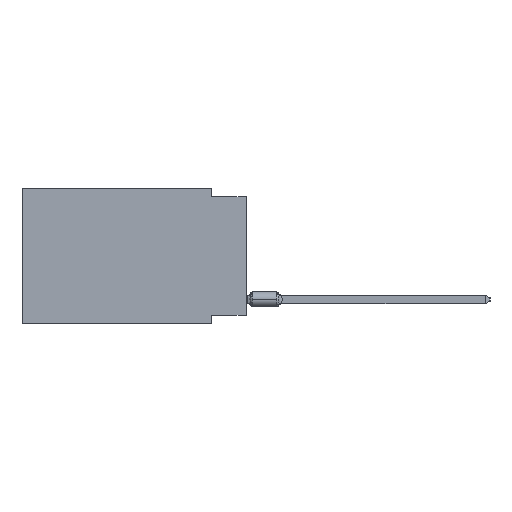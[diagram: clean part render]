
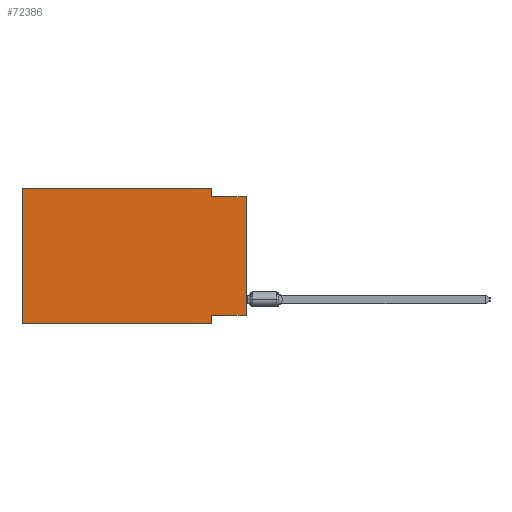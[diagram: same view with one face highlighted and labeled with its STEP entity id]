
A CAD part, left-side view. The second image highlights one B-rep face of the part: STEP entity #72386.
In plain terms, the highlighted planar face has unit normal (-1, 0, 0).
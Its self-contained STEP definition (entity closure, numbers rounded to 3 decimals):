
#480 = EDGE_CURVE ( 'NONE', #50530, #59413, #16337, .T. ) ;
#1245 = VERTEX_POINT ( 'NONE', #71798 ) ;
#3922 = VECTOR ( 'NONE', #43451, 1000. ) ;
#4442 = DIRECTION ( 'NONE',  ( 0., -1., 0. ) ) ;
#7585 = DIRECTION ( 'NONE',  ( 0., 1., 0. ) ) ;
#7791 = VECTOR ( 'NONE', #7585, 1000. ) ;
#11571 = CARTESIAN_POINT ( 'NONE',  ( 0., 16.383, -9.906 ) ) ;
#12327 = PLANE ( 'NONE',  #35123 ) ;
#13555 = CARTESIAN_POINT ( 'NONE',  ( 0., 16.383, -9.906 ) ) ;
#14518 = DIRECTION ( 'NONE',  ( 0., 0., 1. ) ) ;
#15463 = CARTESIAN_POINT ( 'NONE',  ( 0., 16.383, 0. ) ) ;
#16337 = LINE ( 'NONE', #63091, #64548 ) ;
#17380 = CARTESIAN_POINT ( 'NONE',  ( 0., 16.383, 0. ) ) ;
#17696 = EDGE_CURVE ( 'NONE', #68012, #49592, #25215, .T. ) ;
#18709 = CARTESIAN_POINT ( 'NONE',  ( 0., 0., -9.271 ) ) ;
#20062 = CARTESIAN_POINT ( 'NONE',  ( 0., 2.54, -9.906 ) ) ;
#20744 = CARTESIAN_POINT ( 'NONE',  ( 0., 2.54, -9.271 ) ) ;
#21152 = VECTOR ( 'NONE', #14518, 1000. ) ;
#22748 = DIRECTION ( 'NONE',  ( 0., -1., 0. ) ) ;
#22846 = ORIENTED_EDGE ( 'NONE', *, *, #22960, .T. ) ;
#22960 = EDGE_CURVE ( 'NONE', #47992, #1245, #29202, .T. ) ;
#25215 = LINE ( 'NONE', #18709, #7791 ) ;
#25536 = LINE ( 'NONE', #48915, #47731 ) ;
#25605 = LINE ( 'NONE', #72354, #75083 ) ;
#25841 = VERTEX_POINT ( 'NONE', #29473 ) ;
#29111 = EDGE_CURVE ( 'NONE', #39695, #25841, #40395, .T. ) ;
#29202 = LINE ( 'NONE', #11571, #71847 ) ;
#29473 = CARTESIAN_POINT ( 'NONE',  ( 0., 2.54, 0. ) ) ;
#31081 = CARTESIAN_POINT ( 'NONE',  ( 0., 2.54, -0.635 ) ) ;
#31616 = ORIENTED_EDGE ( 'NONE', *, *, #41038, .T. ) ;
#31671 = ORIENTED_EDGE ( 'NONE', *, *, #480, .F. ) ;
#33798 = ORIENTED_EDGE ( 'NONE', *, *, #29111, .F. ) ;
#35123 = AXIS2_PLACEMENT_3D ( 'NONE', #70969, #59468, #35718 ) ;
#35718 = DIRECTION ( 'NONE',  ( 0., 0., -1. ) ) ;
#37394 = VECTOR ( 'NONE', #22748, 1000. ) ;
#39695 = VERTEX_POINT ( 'NONE', #15463 ) ;
#39713 = EDGE_CURVE ( 'NONE', #49592, #1245, #72571, .T. ) ;
#40395 = LINE ( 'NONE', #17380, #37394 ) ;
#40529 = EDGE_CURVE ( 'NONE', #47992, #39695, #61673, .T. ) ;
#41038 = EDGE_CURVE ( 'NONE', #68012, #59413, #25536, .T. ) ;
#43451 = DIRECTION ( 'NONE',  ( 0., 0., -1. ) ) ;
#45725 = DIRECTION ( 'NONE',  ( 0., -1., 0. ) ) ;
#46124 = ORIENTED_EDGE ( 'NONE', *, *, #56951, .F. ) ;
#46616 = ORIENTED_EDGE ( 'NONE', *, *, #17696, .F. ) ;
#47731 = VECTOR ( 'NONE', #49302, 1000. ) ;
#47992 = VERTEX_POINT ( 'NONE', #13555 ) ;
#48915 = CARTESIAN_POINT ( 'NONE',  ( 0., 0., 0. ) ) ;
#48981 = DIRECTION ( 'NONE',  ( 0., 0., -1. ) ) ;
#49302 = DIRECTION ( 'NONE',  ( 0., 0., 1. ) ) ;
#49592 = VERTEX_POINT ( 'NONE', #20744 ) ;
#50530 = VERTEX_POINT ( 'NONE', #31081 ) ;
#55491 = ORIENTED_EDGE ( 'NONE', *, *, #40529, .F. ) ;
#55918 = CARTESIAN_POINT ( 'NONE',  ( 0., 16.383, 0. ) ) ;
#56951 = EDGE_CURVE ( 'NONE', #25841, #50530, #25605, .T. ) ;
#57171 = CARTESIAN_POINT ( 'NONE',  ( 0., 0., -0.635 ) ) ;
#59413 = VERTEX_POINT ( 'NONE', #57171 ) ;
#59468 = DIRECTION ( 'NONE',  ( 1., 0., 0. ) ) ;
#61673 = LINE ( 'NONE', #55918, #21152 ) ;
#62799 = ORIENTED_EDGE ( 'NONE', *, *, #39713, .F. ) ;
#63091 = CARTESIAN_POINT ( 'NONE',  ( 0., 0., -0.635 ) ) ;
#64548 = VECTOR ( 'NONE', #4442, 1000. ) ;
#64839 = FACE_OUTER_BOUND ( 'NONE', #71642, .T. ) ;
#66500 = CARTESIAN_POINT ( 'NONE',  ( 0., 0., -9.271 ) ) ;
#68012 = VERTEX_POINT ( 'NONE', #66500 ) ;
#70969 = CARTESIAN_POINT ( 'NONE',  ( 0., 16.383, 0. ) ) ;
#71642 = EDGE_LOOP ( 'NONE', ( #31616, #31671, #46124, #33798, #55491, #22846, #62799, #46616 ) ) ;
#71798 = CARTESIAN_POINT ( 'NONE',  ( 0., 2.54, -9.906 ) ) ;
#71847 = VECTOR ( 'NONE', #45725, 1000. ) ;
#72354 = CARTESIAN_POINT ( 'NONE',  ( 0., 2.54, 0. ) ) ;
#72386 = ADVANCED_FACE ( 'NONE', ( #64839 ), #12327, .F. ) ;
#72571 = LINE ( 'NONE', #20062, #3922 ) ;
#75083 = VECTOR ( 'NONE', #48981, 1000. ) ;
